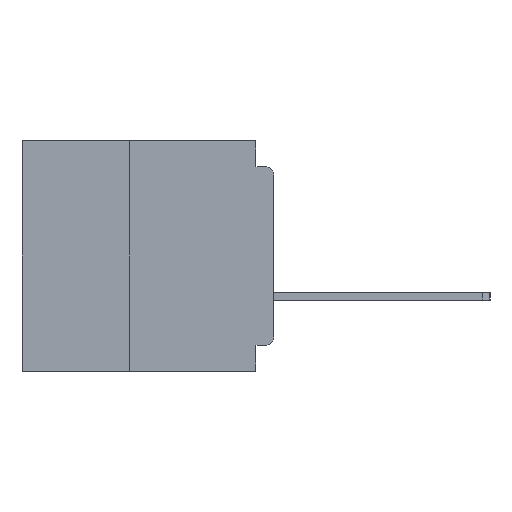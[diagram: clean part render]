
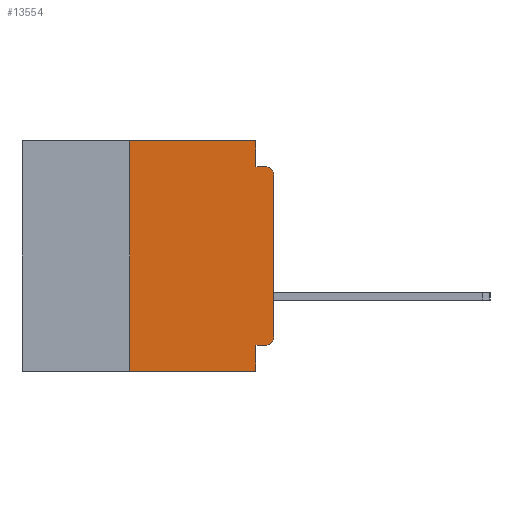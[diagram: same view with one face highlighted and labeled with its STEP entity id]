
A CAD part, left-side view. The second image highlights one B-rep face of the part: STEP entity #13554.
In plain terms, the highlighted planar face has unit normal (-1, 0, 0).
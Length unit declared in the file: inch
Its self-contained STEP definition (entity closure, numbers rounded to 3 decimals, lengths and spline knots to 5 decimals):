
#1552 = DIRECTION ( 'NONE',  ( 1., 0., 0. ) ) ;
#2580 = EDGE_CURVE ( 'NONE', #50902, #52196, #59442, .T. ) ;
#2780 = EDGE_CURVE ( 'NONE', #10549, #58835, #21745, .T. ) ;
#3835 = CARTESIAN_POINT ( 'NONE',  ( 0., 0.437, -0.4 ) ) ;
#5706 = VECTOR ( 'NONE', #13946, 39.37008 ) ;
#8638 = LINE ( 'NONE', #9192, #5706 ) ;
#8906 = EDGE_CURVE ( 'NONE', #34034, #23895, #28888, .T. ) ;
#9192 = CARTESIAN_POINT ( 'NONE',  ( 0., 0., -0.355 ) ) ;
#10102 = VECTOR ( 'NONE', #59704, 39.37008 ) ;
#10549 = VERTEX_POINT ( 'NONE', #15097 ) ;
#11285 = DIRECTION ( 'NONE',  ( 0., 0., 1. ) ) ;
#11360 = CARTESIAN_POINT ( 'NONE',  ( 0., 0.031, -0.4 ) ) ;
#11542 = CARTESIAN_POINT ( 'NONE',  ( 0., 0.25, -0.4 ) ) ;
#11895 = ORIENTED_EDGE ( 'NONE', *, *, #2780, .F. ) ;
#13554 = ADVANCED_FACE ( 'NONE', ( #41903 ), #57314, .F. ) ;
#13888 = CARTESIAN_POINT ( 'NONE',  ( 0., 0.015, -0.06 ) ) ;
#13946 = DIRECTION ( 'NONE',  ( 0., 1., 0. ) ) ;
#14314 = ORIENTED_EDGE ( 'NONE', *, *, #28370, .T. ) ;
#15097 = CARTESIAN_POINT ( 'NONE',  ( 0., 0.25, -0.4 ) ) ;
#15328 = CARTESIAN_POINT ( 'NONE',  ( 0., 0.437, 0. ) ) ;
#15498 = ORIENTED_EDGE ( 'NONE', *, *, #48118, .T. ) ;
#16919 = DIRECTION ( 'NONE',  ( 0., -1., 0. ) ) ;
#17520 = CARTESIAN_POINT ( 'NONE',  ( 0., 0.015, -0.355 ) ) ;
#18595 = DIRECTION ( 'NONE',  ( 0., 0., -1. ) ) ;
#18914 = ORIENTED_EDGE ( 'NONE', *, *, #8906, .F. ) ;
#19567 = CARTESIAN_POINT ( 'NONE',  ( 0., 0.031, -0.4 ) ) ;
#19696 = VERTEX_POINT ( 'NONE', #27394 ) ;
#19746 = CARTESIAN_POINT ( 'NONE',  ( 0., 0.031, -0.045 ) ) ;
#20986 = DIRECTION ( 'NONE',  ( -1., 0., 0. ) ) ;
#21534 = CARTESIAN_POINT ( 'NONE',  ( 0., 0., 0. ) ) ;
#21745 = LINE ( 'NONE', #11542, #57258 ) ;
#22578 = LINE ( 'NONE', #3835, #10102 ) ;
#22971 = DIRECTION ( 'NONE',  ( 0., 0., -1. ) ) ;
#23278 = CARTESIAN_POINT ( 'NONE',  ( 0., 0.031, 0. ) ) ;
#23895 = VERTEX_POINT ( 'NONE', #19567 ) ;
#25333 = LINE ( 'NONE', #21534, #36188 ) ;
#25967 = EDGE_CURVE ( 'NONE', #28871, #34034, #8638, .T. ) ;
#26057 = DIRECTION ( 'NONE',  ( 0., -1., 0. ) ) ;
#26204 = DIRECTION ( 'NONE',  ( 0., 0., 1. ) ) ;
#26259 = CARTESIAN_POINT ( 'NONE',  ( 0., 0.437, 0. ) ) ;
#26370 = LINE ( 'NONE', #26259, #27847 ) ;
#27394 = CARTESIAN_POINT ( 'NONE',  ( 0., 0., -0.06 ) ) ;
#27440 = VECTOR ( 'NONE', #57869, 39.37008 ) ;
#27847 = VECTOR ( 'NONE', #26057, 39.37008 ) ;
#28370 = EDGE_CURVE ( 'NONE', #10549, #23895, #22578, .T. ) ;
#28871 = VERTEX_POINT ( 'NONE', #17520 ) ;
#28888 = LINE ( 'NONE', #11360, #27440 ) ;
#31395 = CARTESIAN_POINT ( 'NONE',  ( 0., 0., -0.34 ) ) ;
#31737 = ORIENTED_EDGE ( 'NONE', *, *, #25967, .F. ) ;
#31879 = AXIS2_PLACEMENT_3D ( 'NONE', #15328, #1552, #34227 ) ;
#32704 = EDGE_CURVE ( 'NONE', #52196, #42907, #46717, .T. ) ;
#32948 = ORIENTED_EDGE ( 'NONE', *, *, #2580, .F. ) ;
#34034 = VERTEX_POINT ( 'NONE', #40731 ) ;
#34227 = DIRECTION ( 'NONE',  ( 0., 0., -1. ) ) ;
#34495 = AXIS2_PLACEMENT_3D ( 'NONE', #48753, #20986, #53432 ) ;
#34740 = EDGE_CURVE ( 'NONE', #28871, #56023, #46836, .T. ) ;
#36188 = VECTOR ( 'NONE', #26204, 39.37008 ) ;
#38054 = ORIENTED_EDGE ( 'NONE', *, *, #32704, .F. ) ;
#39048 = ORIENTED_EDGE ( 'NONE', *, *, #45346, .T. ) ;
#40731 = CARTESIAN_POINT ( 'NONE',  ( 0., 0.031, -0.355 ) ) ;
#41903 = FACE_OUTER_BOUND ( 'NONE', #52550, .T. ) ;
#42907 = VERTEX_POINT ( 'NONE', #50299 ) ;
#44708 = CARTESIAN_POINT ( 'NONE',  ( 0., 0., -0.045 ) ) ;
#45346 = EDGE_CURVE ( 'NONE', #19696, #42907, #53265, .T. ) ;
#45781 = EDGE_CURVE ( 'NONE', #58835, #50902, #26370, .T. ) ;
#46378 = DIRECTION ( 'NONE',  ( -1., 0., 0. ) ) ;
#46717 = LINE ( 'NONE', #44708, #48152 ) ;
#46814 = AXIS2_PLACEMENT_3D ( 'NONE', #13888, #46378, #18595 ) ;
#46836 = CIRCLE ( 'NONE', #34495, 0.015 ) ;
#48118 = EDGE_CURVE ( 'NONE', #56023, #19696, #25333, .T. ) ;
#48152 = VECTOR ( 'NONE', #16919, 39.37008 ) ;
#48753 = CARTESIAN_POINT ( 'NONE',  ( 0., 0.015, -0.34 ) ) ;
#50299 = CARTESIAN_POINT ( 'NONE',  ( 0., 0.015, -0.045 ) ) ;
#50648 = CARTESIAN_POINT ( 'NONE',  ( 0., 0.25, 0. ) ) ;
#50902 = VERTEX_POINT ( 'NONE', #51584 ) ;
#51584 = CARTESIAN_POINT ( 'NONE',  ( 0., 0.031, 0. ) ) ;
#52196 = VERTEX_POINT ( 'NONE', #19746 ) ;
#52550 = EDGE_LOOP ( 'NONE', ( #15498, #39048, #38054, #32948, #58675, #11895, #14314, #18914, #31737, #54769 ) ) ;
#53265 = CIRCLE ( 'NONE', #46814, 0.015 ) ;
#53432 = DIRECTION ( 'NONE',  ( 0., 0., -1. ) ) ;
#54769 = ORIENTED_EDGE ( 'NONE', *, *, #34740, .T. ) ;
#56023 = VERTEX_POINT ( 'NONE', #31395 ) ;
#57258 = VECTOR ( 'NONE', #11285, 39.37008 ) ;
#57314 = PLANE ( 'NONE',  #31879 ) ;
#57869 = DIRECTION ( 'NONE',  ( 0., 0., -1. ) ) ;
#58011 = VECTOR ( 'NONE', #22971, 39.37008 ) ;
#58675 = ORIENTED_EDGE ( 'NONE', *, *, #45781, .F. ) ;
#58835 = VERTEX_POINT ( 'NONE', #50648 ) ;
#59442 = LINE ( 'NONE', #23278, #58011 ) ;
#59704 = DIRECTION ( 'NONE',  ( 0., -1., 0. ) ) ;
